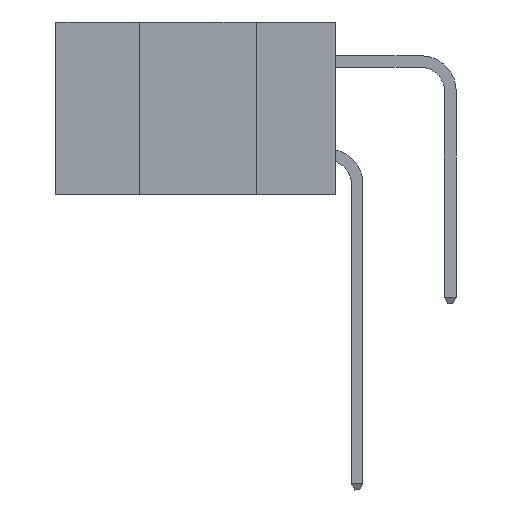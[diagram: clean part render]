
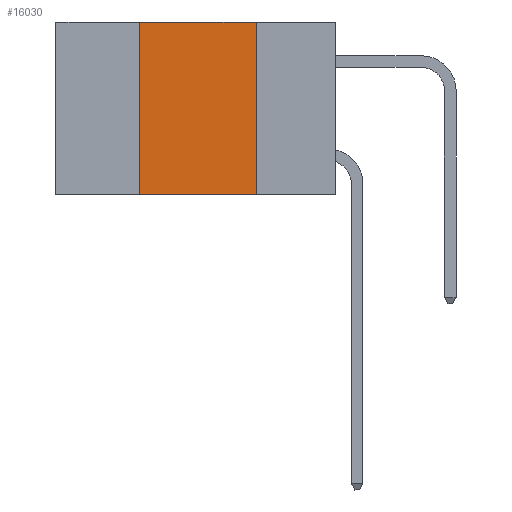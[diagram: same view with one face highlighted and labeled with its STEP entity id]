
A CAD part, left-side view. The second image highlights one B-rep face of the part: STEP entity #16030.
In plain terms, the highlighted planar face has unit normal (-1, 0, 0).
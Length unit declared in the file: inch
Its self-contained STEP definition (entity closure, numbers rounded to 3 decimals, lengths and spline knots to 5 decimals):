
#1941 = CARTESIAN_POINT ( 'NONE',  ( 0., 0.6, 0. ) ) ;
#4166 = CARTESIAN_POINT ( 'NONE',  ( 0., 0.42, 0. ) ) ;
#4428 = CARTESIAN_POINT ( 'NONE',  ( 0., 0.42, 0. ) ) ;
#4707 = VECTOR ( 'NONE', #9301, 39.37008 ) ;
#7684 = DIRECTION ( 'NONE',  ( 0., 0., -1. ) ) ;
#8271 = VECTOR ( 'NONE', #23738, 39.37008 ) ;
#9301 = DIRECTION ( 'NONE',  ( 0., 0., -1. ) ) ;
#10283 = LINE ( 'NONE', #16548, #4707 ) ;
#10447 = CARTESIAN_POINT ( 'NONE',  ( 0., 0.17, -0.37 ) ) ;
#10537 = ORIENTED_EDGE ( 'NONE', *, *, #19421, .T. ) ;
#10551 = VERTEX_POINT ( 'NONE', #17655 ) ;
#12043 = VECTOR ( 'NONE', #19272, 39.37008 ) ;
#12294 = CARTESIAN_POINT ( 'NONE',  ( 0., 0.17, 0. ) ) ;
#12332 = ORIENTED_EDGE ( 'NONE', *, *, #17570, .F. ) ;
#12348 = DIRECTION ( 'NONE',  ( 0., -1., 0. ) ) ;
#12636 = FACE_OUTER_BOUND ( 'NONE', #15745, .T. ) ;
#13451 = LINE ( 'NONE', #17742, #17226 ) ;
#13858 = LINE ( 'NONE', #18209, #8271 ) ;
#15703 = EDGE_CURVE ( 'NONE', #18884, #22691, #10283, .T. ) ;
#15745 = EDGE_LOOP ( 'NONE', ( #17568, #12332, #20806, #10537 ) ) ;
#16030 = ADVANCED_FACE ( 'NONE', ( #12636 ), #22930, .F. ) ;
#16548 = CARTESIAN_POINT ( 'NONE',  ( 0., 0.17, 0. ) ) ;
#17005 = LINE ( 'NONE', #4166, #12043 ) ;
#17011 = DIRECTION ( 'NONE',  ( 1., 0., 0. ) ) ;
#17226 = VECTOR ( 'NONE', #12348, 39.37008 ) ;
#17568 = ORIENTED_EDGE ( 'NONE', *, *, #15703, .F. ) ;
#17570 = EDGE_CURVE ( 'NONE', #18032, #18884, #13451, .T. ) ;
#17655 = CARTESIAN_POINT ( 'NONE',  ( 0., 0.42, -0.37 ) ) ;
#17742 = CARTESIAN_POINT ( 'NONE',  ( 0., 0.6, 0. ) ) ;
#18032 = VERTEX_POINT ( 'NONE', #4428 ) ;
#18209 = CARTESIAN_POINT ( 'NONE',  ( 0., 0.6, -0.37 ) ) ;
#18884 = VERTEX_POINT ( 'NONE', #12294 ) ;
#19272 = DIRECTION ( 'NONE',  ( 0., 0., 1. ) ) ;
#19421 = EDGE_CURVE ( 'NONE', #10551, #22691, #13858, .T. ) ;
#19869 = EDGE_CURVE ( 'NONE', #10551, #18032, #17005, .T. ) ;
#20639 = AXIS2_PLACEMENT_3D ( 'NONE', #1941, #17011, #7684 ) ;
#20806 = ORIENTED_EDGE ( 'NONE', *, *, #19869, .F. ) ;
#22691 = VERTEX_POINT ( 'NONE', #10447 ) ;
#22930 = PLANE ( 'NONE',  #20639 ) ;
#23738 = DIRECTION ( 'NONE',  ( 0., -1., 0. ) ) ;
